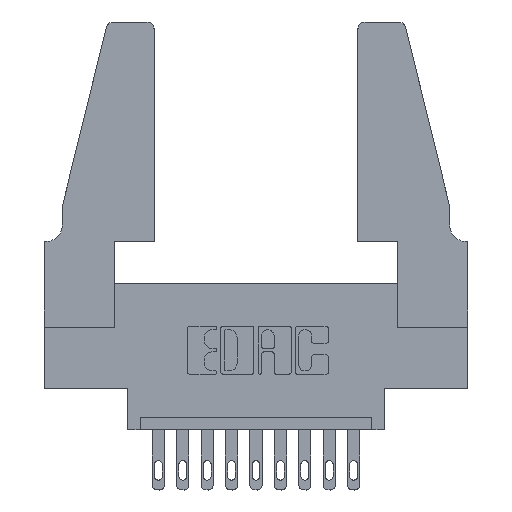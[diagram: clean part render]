
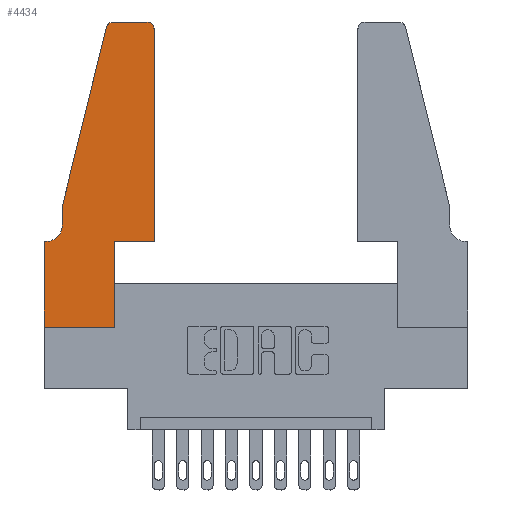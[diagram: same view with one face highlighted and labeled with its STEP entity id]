
A CAD part, top view. The second image highlights one B-rep face of the part: STEP entity #4434.
In plain terms, the highlighted planar face has unit normal (0, 0, 1).
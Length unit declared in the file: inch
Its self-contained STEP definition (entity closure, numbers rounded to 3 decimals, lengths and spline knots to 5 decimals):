
#83 = LINE ( 'NONE', #8038, #3032 ) ;
#87 = CARTESIAN_POINT ( 'NONE',  ( 0., 0.35, 0.37 ) ) ;
#145 = VERTEX_POINT ( 'NONE', #11576 ) ;
#153 = FACE_OUTER_BOUND ( 'NONE', #5770, .T. ) ;
#199 = DIRECTION ( 'NONE',  ( 1., 0., 0. ) ) ;
#207 = DIRECTION ( 'NONE',  ( 0., 1., 0. ) ) ;
#212 = DIRECTION ( 'NONE',  ( 0., 0., 1. ) ) ;
#334 = CARTESIAN_POINT ( 'NONE',  ( 0.4505, 0.35, 0.37 ) ) ;
#427 = EDGE_CURVE ( 'NONE', #7912, #10538, #6246, .T. ) ;
#543 = VERTEX_POINT ( 'NONE', #87 ) ;
#654 = LINE ( 'NONE', #3869, #8523 ) ;
#726 = VECTOR ( 'NONE', #199, 39.37008 ) ;
#962 = EDGE_CURVE ( 'NONE', #7879, #543, #12919, .T. ) ;
#1116 = ORIENTED_EDGE ( 'NONE', *, *, #7731, .T. ) ;
#1267 = EDGE_CURVE ( 'NONE', #6941, #145, #4778, .T. ) ;
#1279 = DIRECTION ( 'NONE',  ( 0., 1., 0. ) ) ;
#1476 = ORIENTED_EDGE ( 'NONE', *, *, #9176, .T. ) ;
#1650 = ORIENTED_EDGE ( 'NONE', *, *, #6727, .T. ) ;
#1690 = DIRECTION ( 'NONE',  ( 0., -1., 0. ) ) ;
#1874 = ORIENTED_EDGE ( 'NONE', *, *, #1267, .T. ) ;
#1933 = EDGE_CURVE ( 'NONE', #10219, #8969, #8594, .T. ) ;
#2307 = DIRECTION ( 'NONE',  ( 0., 0., 1. ) ) ;
#2774 = VERTEX_POINT ( 'NONE', #12562 ) ;
#2903 = VECTOR ( 'NONE', #207, 39.37008 ) ;
#3032 = VECTOR ( 'NONE', #11178, 39.37008 ) ;
#3128 = CARTESIAN_POINT ( 'NONE',  ( 0.284, 1.25, 0.37 ) ) ;
#3175 = DIRECTION ( 'NONE',  ( 0., 0., -1. ) ) ;
#3263 = CARTESIAN_POINT ( 'NONE',  ( 0., 0., 0.37 ) ) ;
#3279 = CARTESIAN_POINT ( 'NONE',  ( 0., 0.35, 0.37 ) ) ;
#3581 = VERTEX_POINT ( 'NONE', #6419 ) ;
#3727 = ORIENTED_EDGE ( 'NONE', *, *, #1933, .T. ) ;
#3869 = CARTESIAN_POINT ( 'NONE',  ( 0.0755, 0.5, 0.37 ) ) ;
#4150 = AXIS2_PLACEMENT_3D ( 'NONE', #3279, #10523, #5348 ) ;
#4286 = DIRECTION ( 'NONE',  ( 0., -1., 0. ) ) ;
#4321 = VECTOR ( 'NONE', #10939, 39.37008 ) ;
#4434 = ADVANCED_FACE ( 'NONE', ( #153 ), #8370, .T. ) ;
#4479 = ORIENTED_EDGE ( 'NONE', *, *, #962, .T. ) ;
#4532 = CARTESIAN_POINT ( 'NONE',  ( 0.2865, 0.35, 0.37 ) ) ;
#4774 = VERTEX_POINT ( 'NONE', #11258 ) ;
#4778 = CIRCLE ( 'NONE', #11940, 0.03 ) ;
#5067 = CIRCLE ( 'NONE', #8936, 0.03 ) ;
#5303 = ORIENTED_EDGE ( 'NONE', *, *, #13005, .T. ) ;
#5304 = LINE ( 'NONE', #10797, #4321 ) ;
#5348 = DIRECTION ( 'NONE',  ( 1., 0., 0. ) ) ;
#5405 = AXIS2_PLACEMENT_3D ( 'NONE', #9336, #3175, #11477 ) ;
#5440 = EDGE_CURVE ( 'NONE', #10538, #10219, #7530, .T. ) ;
#5770 = EDGE_LOOP ( 'NONE', ( #1650, #1874, #10734, #7864, #1116, #4479, #10655, #9064, #7929, #3727, #5303, #1476 ) ) ;
#5990 = CARTESIAN_POINT ( 'NONE',  ( 0., 0., 0.37 ) ) ;
#6246 = LINE ( 'NONE', #8932, #6876 ) ;
#6419 = CARTESIAN_POINT ( 'NONE',  ( 0.0755, 0.5, 0.37 ) ) ;
#6727 = EDGE_CURVE ( 'NONE', #4774, #6941, #83, .T. ) ;
#6876 = VECTOR ( 'NONE', #8892, 39.37008 ) ;
#6941 = VERTEX_POINT ( 'NONE', #3128 ) ;
#7114 = VERTEX_POINT ( 'NONE', #11847 ) ;
#7530 = LINE ( 'NONE', #4532, #2903 ) ;
#7731 = EDGE_CURVE ( 'NONE', #2774, #7879, #12437, .T. ) ;
#7818 = VECTOR ( 'NONE', #10197, 39.37008 ) ;
#7864 = ORIENTED_EDGE ( 'NONE', *, *, #10314, .T. ) ;
#7879 = VERTEX_POINT ( 'NONE', #8373 ) ;
#7912 = VERTEX_POINT ( 'NONE', #5990 ) ;
#7929 = ORIENTED_EDGE ( 'NONE', *, *, #5440, .T. ) ;
#8038 = CARTESIAN_POINT ( 'NONE',  ( 0.2605, 1.25, 0.37 ) ) ;
#8370 = PLANE ( 'NONE',  #4150 ) ;
#8373 = CARTESIAN_POINT ( 'NONE',  ( 0.0055, 0.35, 0.37 ) ) ;
#8523 = VECTOR ( 'NONE', #1690, 39.37008 ) ;
#8551 = CARTESIAN_POINT ( 'NONE',  ( 0.4505, 0.35, 0.37 ) ) ;
#8594 = LINE ( 'NONE', #334, #726 ) ;
#8892 = DIRECTION ( 'NONE',  ( 1., 0., 0. ) ) ;
#8932 = CARTESIAN_POINT ( 'NONE',  ( 0., 0., 0.37 ) ) ;
#8936 = AXIS2_PLACEMENT_3D ( 'NONE', #10670, #212, #10629 ) ;
#8969 = VERTEX_POINT ( 'NONE', #13390 ) ;
#9064 = ORIENTED_EDGE ( 'NONE', *, *, #427, .T. ) ;
#9122 = VECTOR ( 'NONE', #1279, 39.37008 ) ;
#9176 = EDGE_CURVE ( 'NONE', #7114, #4774, #5067, .T. ) ;
#9336 = CARTESIAN_POINT ( 'NONE',  ( 0.0055, 0.42, 0.37 ) ) ;
#9853 = CARTESIAN_POINT ( 'NONE',  ( 0.2865, 0., 0.37 ) ) ;
#10197 = DIRECTION ( 'NONE',  ( -1., 0., 0. ) ) ;
#10219 = VERTEX_POINT ( 'NONE', #11846 ) ;
#10279 = CARTESIAN_POINT ( 'NONE',  ( 0.284, 1.22, 0.37 ) ) ;
#10314 = EDGE_CURVE ( 'NONE', #3581, #2774, #654, .T. ) ;
#10331 = CARTESIAN_POINT ( 'NONE',  ( 0.0755, 0.35, 0.37 ) ) ;
#10432 = EDGE_CURVE ( 'NONE', #543, #7912, #12988, .T. ) ;
#10454 = DIRECTION ( 'NONE',  ( 1., 0., 0. ) ) ;
#10523 = DIRECTION ( 'NONE',  ( 0., 0., 1. ) ) ;
#10538 = VERTEX_POINT ( 'NONE', #9853 ) ;
#10629 = DIRECTION ( 'NONE',  ( 1., 0., 0. ) ) ;
#10655 = ORIENTED_EDGE ( 'NONE', *, *, #10432, .T. ) ;
#10670 = CARTESIAN_POINT ( 'NONE',  ( 0.4205, 1.22, 0.37 ) ) ;
#10734 = ORIENTED_EDGE ( 'NONE', *, *, #11632, .T. ) ;
#10797 = CARTESIAN_POINT ( 'NONE',  ( 0.0755, 0.5, 0.37 ) ) ;
#10939 = DIRECTION ( 'NONE',  ( -0.239, -0.971, 0. ) ) ;
#10942 = LINE ( 'NONE', #8551, #9122 ) ;
#11178 = DIRECTION ( 'NONE',  ( -1., 0., 0. ) ) ;
#11258 = CARTESIAN_POINT ( 'NONE',  ( 0.4205, 1.25, 0.37 ) ) ;
#11477 = DIRECTION ( 'NONE',  ( -1., 0., 0. ) ) ;
#11576 = CARTESIAN_POINT ( 'NONE',  ( 0.25487, 1.22718, 0.37 ) ) ;
#11632 = EDGE_CURVE ( 'NONE', #145, #3581, #5304, .T. ) ;
#11846 = CARTESIAN_POINT ( 'NONE',  ( 0.2865, 0.35, 0.37 ) ) ;
#11847 = CARTESIAN_POINT ( 'NONE',  ( 0.4505, 1.22, 0.37 ) ) ;
#11940 = AXIS2_PLACEMENT_3D ( 'NONE', #10279, #2307, #10454 ) ;
#12020 = VECTOR ( 'NONE', #4286, 39.37008 ) ;
#12437 = CIRCLE ( 'NONE', #5405, 0.07 ) ;
#12562 = CARTESIAN_POINT ( 'NONE',  ( 0.0755, 0.42, 0.37 ) ) ;
#12919 = LINE ( 'NONE', #10331, #7818 ) ;
#12988 = LINE ( 'NONE', #3263, #12020 ) ;
#13005 = EDGE_CURVE ( 'NONE', #8969, #7114, #10942, .T. ) ;
#13390 = CARTESIAN_POINT ( 'NONE',  ( 0.4505, 0.35, 0.37 ) ) ;
